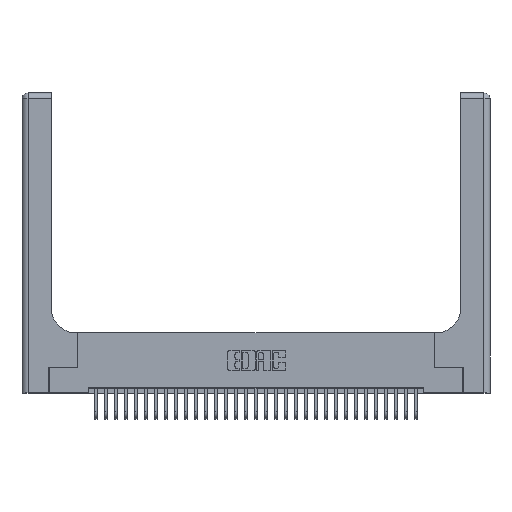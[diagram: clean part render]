
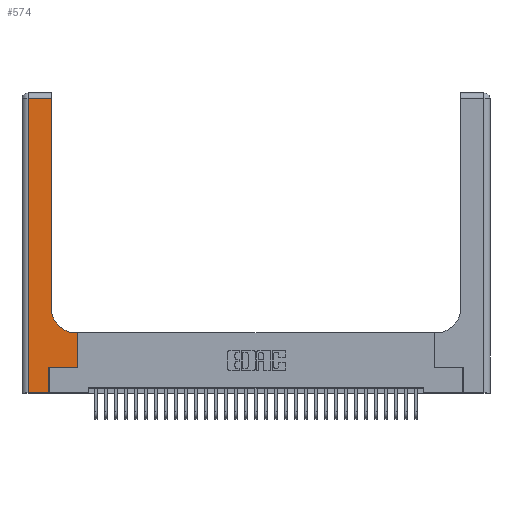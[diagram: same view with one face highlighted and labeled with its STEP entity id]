
A CAD part, top view. The second image highlights one B-rep face of the part: STEP entity #574.
In plain terms, the highlighted planar face has unit normal (0, 0, 1).
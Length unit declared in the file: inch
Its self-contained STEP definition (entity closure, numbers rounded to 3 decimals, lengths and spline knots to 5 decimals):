
#414 = ORIENTED_EDGE ( 'NONE', *, *, #16215, .T. ) ;
#574 = ADVANCED_FACE ( 'NONE', ( #30389 ), #11409, .F. ) ;
#826 = CARTESIAN_POINT ( 'NONE',  ( 0., 0., 0.37 ) ) ;
#1713 = LINE ( 'NONE', #23647, #14104 ) ;
#2865 = LINE ( 'NONE', #20139, #19334 ) ;
#2975 = CARTESIAN_POINT ( 'NONE',  ( 0.2915, 0.6, 0.37 ) ) ;
#3543 = VERTEX_POINT ( 'NONE', #29337 ) ;
#3840 = LINE ( 'NONE', #2975, #23228 ) ;
#5654 = AXIS2_PLACEMENT_3D ( 'NONE', #28090, #30476, #16267 ) ;
#6381 = EDGE_CURVE ( 'NONE', #26241, #29327, #1713, .T. ) ;
#6657 = ORIENTED_EDGE ( 'NONE', *, *, #18719, .T. ) ;
#7245 = CARTESIAN_POINT ( 'NONE',  ( 0.5415, 0.6, 0.37 ) ) ;
#7342 = AXIS2_PLACEMENT_3D ( 'NONE', #12877, #29517, #15300 ) ;
#7542 = VECTOR ( 'NONE', #28117, 39.37008 ) ;
#7974 = DIRECTION ( 'NONE',  ( -1., 0., 0. ) ) ;
#8299 = CARTESIAN_POINT ( 'NONE',  ( 0.06, 3., 0.37 ) ) ;
#8340 = DIRECTION ( 'NONE',  ( 1., 0., 0. ) ) ;
#8489 = VECTOR ( 'NONE', #30329, 39.37008 ) ;
#8604 = VERTEX_POINT ( 'NONE', #12223 ) ;
#8740 = VECTOR ( 'NONE', #9614, 39.37008 ) ;
#8855 = EDGE_CURVE ( 'NONE', #15787, #3543, #16199, .T. ) ;
#9570 = ORIENTED_EDGE ( 'NONE', *, *, #20473, .T. ) ;
#9614 = DIRECTION ( 'NONE',  ( 0., 1., 0. ) ) ;
#9721 = VERTEX_POINT ( 'NONE', #26155 ) ;
#10186 = EDGE_CURVE ( 'NONE', #29327, #20586, #3840, .T. ) ;
#10499 = ORIENTED_EDGE ( 'NONE', *, *, #6381, .T. ) ;
#11409 = PLANE ( 'NONE',  #5654 ) ;
#11691 = DIRECTION ( 'NONE',  ( 0., 1., 0. ) ) ;
#11978 = CARTESIAN_POINT ( 'NONE',  ( 0.269, 0., 0.37 ) ) ;
#12223 = CARTESIAN_POINT ( 'NONE',  ( 0.2915, 0.85, 0.37 ) ) ;
#12447 = ORIENTED_EDGE ( 'NONE', *, *, #19595, .T. ) ;
#12877 = CARTESIAN_POINT ( 'NONE',  ( 0.5415, 0.85, 0.37 ) ) ;
#13187 = ORIENTED_EDGE ( 'NONE', *, *, #29205, .T. ) ;
#13356 = ORIENTED_EDGE ( 'NONE', *, *, #8855, .T. ) ;
#13700 = CARTESIAN_POINT ( 'NONE',  ( 0.2915, 3., 0.37 ) ) ;
#13762 = EDGE_CURVE ( 'NONE', #26542, #15787, #15537, .T. ) ;
#13962 = VERTEX_POINT ( 'NONE', #28299 ) ;
#14104 = VECTOR ( 'NONE', #11691, 39.37008 ) ;
#14773 = VECTOR ( 'NONE', #22770, 39.37008 ) ;
#15248 = LINE ( 'NONE', #11978, #8740 ) ;
#15300 = DIRECTION ( 'NONE',  ( 1., 0., 0. ) ) ;
#15537 = LINE ( 'NONE', #8299, #14773 ) ;
#15787 = VERTEX_POINT ( 'NONE', #16968 ) ;
#16199 = LINE ( 'NONE', #826, #23317 ) ;
#16215 = EDGE_CURVE ( 'NONE', #8604, #13962, #26900, .T. ) ;
#16267 = DIRECTION ( 'NONE',  ( -1., 0., 0. ) ) ;
#16968 = CARTESIAN_POINT ( 'NONE',  ( 0.06, 0., 0.37 ) ) ;
#17056 = ORIENTED_EDGE ( 'NONE', *, *, #10186, .T. ) ;
#18719 = EDGE_CURVE ( 'NONE', #3543, #9721, #15248, .T. ) ;
#19334 = VECTOR ( 'NONE', #20038, 39.37008 ) ;
#19595 = EDGE_CURVE ( 'NONE', #13962, #26542, #2865, .T. ) ;
#20038 = DIRECTION ( 'NONE',  ( -1., 0., 0. ) ) ;
#20139 = CARTESIAN_POINT ( 'NONE',  ( 0., 2.94, 0.37 ) ) ;
#20473 = EDGE_CURVE ( 'NONE', #9721, #26241, #26702, .T. ) ;
#20586 = VERTEX_POINT ( 'NONE', #7245 ) ;
#22770 = DIRECTION ( 'NONE',  ( 0., -1., 0. ) ) ;
#23228 = VECTOR ( 'NONE', #7974, 39.37008 ) ;
#23317 = VECTOR ( 'NONE', #8340, 39.37008 ) ;
#23647 = CARTESIAN_POINT ( 'NONE',  ( 0.5585, 0.25, 0.37 ) ) ;
#25768 = CARTESIAN_POINT ( 'NONE',  ( 0.269, 0.25, 0.37 ) ) ;
#26155 = CARTESIAN_POINT ( 'NONE',  ( 0.269, 0.25, 0.37 ) ) ;
#26241 = VERTEX_POINT ( 'NONE', #27901 ) ;
#26542 = VERTEX_POINT ( 'NONE', #27079 ) ;
#26702 = LINE ( 'NONE', #25768, #7542 ) ;
#26900 = LINE ( 'NONE', #13700, #8489 ) ;
#27079 = CARTESIAN_POINT ( 'NONE',  ( 0.06, 2.94, 0.37 ) ) ;
#27480 = CIRCLE ( 'NONE', #7342, 0.25 ) ;
#27641 = CARTESIAN_POINT ( 'NONE',  ( 0.5585, 0.6, 0.37 ) ) ;
#27901 = CARTESIAN_POINT ( 'NONE',  ( 0.5585, 0.25, 0.37 ) ) ;
#28090 = CARTESIAN_POINT ( 'NONE',  ( 0., 3., 0.37 ) ) ;
#28117 = DIRECTION ( 'NONE',  ( 1., 0., 0. ) ) ;
#28299 = CARTESIAN_POINT ( 'NONE',  ( 0.2915, 2.94, 0.37 ) ) ;
#29205 = EDGE_CURVE ( 'NONE', #20586, #8604, #27480, .T. ) ;
#29327 = VERTEX_POINT ( 'NONE', #27641 ) ;
#29337 = CARTESIAN_POINT ( 'NONE',  ( 0.269, 0., 0.37 ) ) ;
#29517 = DIRECTION ( 'NONE',  ( 0., 0., -1. ) ) ;
#29822 = EDGE_LOOP ( 'NONE', ( #414, #12447, #30663, #13356, #6657, #9570, #10499, #17056, #13187 ) ) ;
#30329 = DIRECTION ( 'NONE',  ( 0., 1., 0. ) ) ;
#30389 = FACE_OUTER_BOUND ( 'NONE', #29822, .T. ) ;
#30476 = DIRECTION ( 'NONE',  ( 0., 0., -1. ) ) ;
#30663 = ORIENTED_EDGE ( 'NONE', *, *, #13762, .T. ) ;
